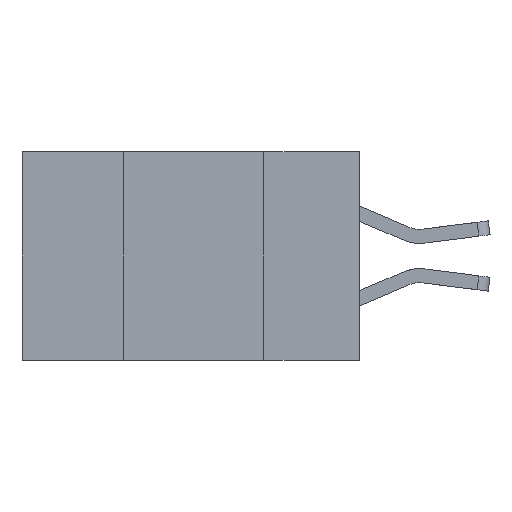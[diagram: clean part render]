
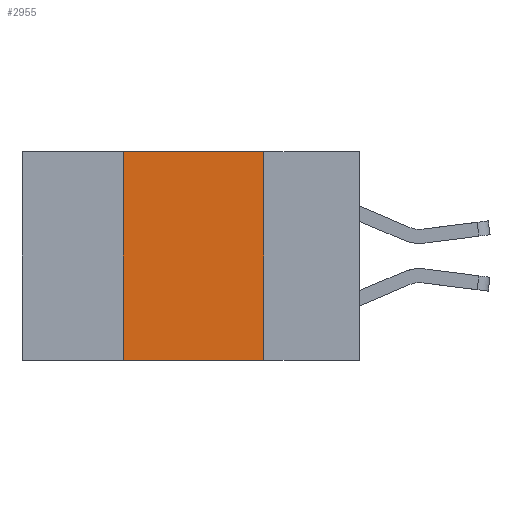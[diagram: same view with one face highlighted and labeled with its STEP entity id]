
A CAD part, left-side view. The second image highlights one B-rep face of the part: STEP entity #2955.
In plain terms, the highlighted planar face has unit normal (-1, 0, 0).
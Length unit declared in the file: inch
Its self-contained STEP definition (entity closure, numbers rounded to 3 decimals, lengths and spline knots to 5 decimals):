
#137 = EDGE_LOOP ( 'NONE', ( #1126, #1413, #1543, #1582 ) ) ;
#987 = DIRECTION ( 'NONE',  ( 0., 0., -1. ) ) ;
#996 = DIRECTION ( 'NONE',  ( 1., 0., 0. ) ) ;
#1102 = VERTEX_POINT ( 'NONE', #11273 ) ;
#1126 = ORIENTED_EDGE ( 'NONE', *, *, #4046, .F. ) ;
#1206 = CARTESIAN_POINT ( 'NONE',  ( 0., 0.6, 0. ) ) ;
#1413 = ORIENTED_EDGE ( 'NONE', *, *, #6490, .F. ) ;
#1543 = ORIENTED_EDGE ( 'NONE', *, *, #7834, .F. ) ;
#1571 = PLANE ( 'NONE',  #1609 ) ;
#1582 = ORIENTED_EDGE ( 'NONE', *, *, #7530, .T. ) ;
#1609 = AXIS2_PLACEMENT_3D ( 'NONE', #1206, #996, #987 ) ;
#1752 = DIRECTION ( 'NONE',  ( 0., -1., 0. ) ) ;
#2190 = VECTOR ( 'NONE', #3982, 39.37008 ) ;
#2413 = CARTESIAN_POINT ( 'NONE',  ( 0., 0.42, -0.37 ) ) ;
#2560 = VECTOR ( 'NONE', #7341, 39.37008 ) ;
#2701 = CARTESIAN_POINT ( 'NONE',  ( 0., 0.6, -0.37 ) ) ;
#2845 = LINE ( 'NONE', #5651, #2560 ) ;
#2955 = ADVANCED_FACE ( 'NONE', ( #9538 ), #1571, .F. ) ;
#3218 = LINE ( 'NONE', #2701, #7634 ) ;
#3423 = CARTESIAN_POINT ( 'NONE',  ( 0., 0.17, 0. ) ) ;
#3721 = VERTEX_POINT ( 'NONE', #2413 ) ;
#3982 = DIRECTION ( 'NONE',  ( 0., 0., 1. ) ) ;
#4046 = EDGE_CURVE ( 'NONE', #11216, #1102, #2845, .T. ) ;
#4889 = CARTESIAN_POINT ( 'NONE',  ( 0., 0.42, 0. ) ) ;
#5651 = CARTESIAN_POINT ( 'NONE',  ( 0., 0.17, 0. ) ) ;
#6490 = EDGE_CURVE ( 'NONE', #6880, #11216, #9613, .T. ) ;
#6880 = VERTEX_POINT ( 'NONE', #9586 ) ;
#7247 = VECTOR ( 'NONE', #8128, 39.37008 ) ;
#7341 = DIRECTION ( 'NONE',  ( 0., 0., -1. ) ) ;
#7530 = EDGE_CURVE ( 'NONE', #3721, #1102, #3218, .T. ) ;
#7634 = VECTOR ( 'NONE', #1752, 39.37008 ) ;
#7834 = EDGE_CURVE ( 'NONE', #3721, #6880, #11510, .T. ) ;
#8128 = DIRECTION ( 'NONE',  ( 0., -1., 0. ) ) ;
#9538 = FACE_OUTER_BOUND ( 'NONE', #137, .T. ) ;
#9586 = CARTESIAN_POINT ( 'NONE',  ( 0., 0.42, 0. ) ) ;
#9613 = LINE ( 'NONE', #9911, #7247 ) ;
#9911 = CARTESIAN_POINT ( 'NONE',  ( 0., 0.6, 0. ) ) ;
#11216 = VERTEX_POINT ( 'NONE', #3423 ) ;
#11273 = CARTESIAN_POINT ( 'NONE',  ( 0., 0.17, -0.37 ) ) ;
#11510 = LINE ( 'NONE', #4889, #2190 ) ;
